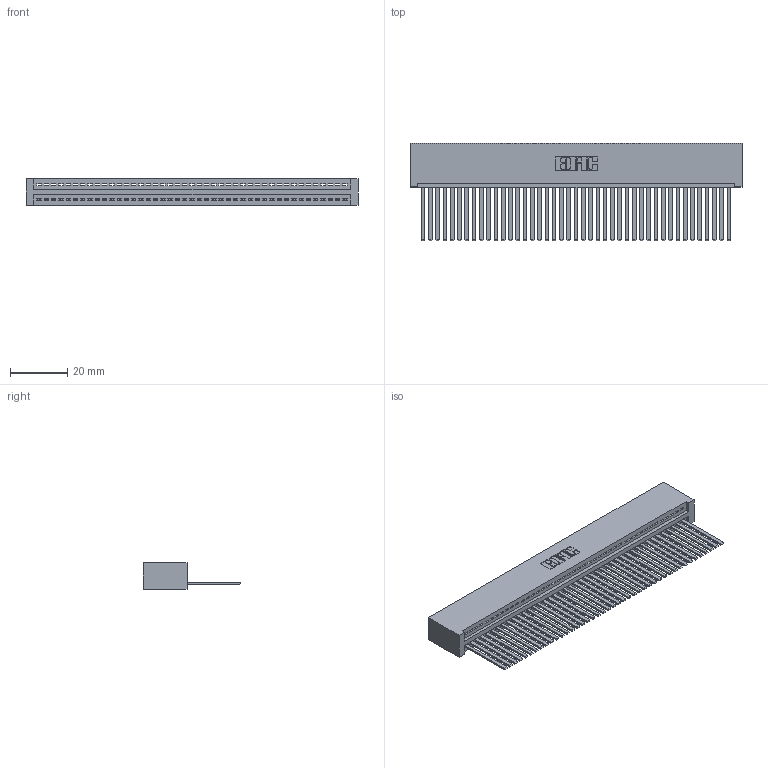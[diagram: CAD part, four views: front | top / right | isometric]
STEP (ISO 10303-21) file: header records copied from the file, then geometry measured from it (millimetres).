
FILE_DESCRIPTION (( 'STEP AP203' ), '1' );
FILE_NAME ('395-043-544-101.STEP', '2019-10-22T14:47:17', ( '' ), ( '' ), 'SwSTEP 2.0', 'SolidWorks 2016', '' );
FILE_SCHEMA (( 'CONFIG_CONTROL_DESIGN' ));
Length unit declared in the file: inch
Products named in the file (3): 345-292-001_345-293-144; 395-043-544-101; 345 Part_No Mounting Lugs
Assembly tree (44 placements, depth 2):
  395-043-544-101
    345 Part_No Mounting Lugs
    345-292-001_345-293-144  x43
Bounding box: 115.82 x 33.96 x 9.4 mm (x, y, z)
Volume: 12091.6 mm3; surface area: 17767.5 mm2
Topology: 44 solids, 44 shells, 2354 faces, 7111 edges, 4682 vertices
Faces by surface type: plane 1624, cylinder 730
Entity records: 31767 total; most frequent: CARTESIAN_POINT 5509, ORIENTED_EDGE 5486, DIRECTION 4801, EDGE_CURVE 2743, LINE 2451, VECTOR 2451, VERTEX_POINT 1826, AXIS2_PLACEMENT_3D 1175
